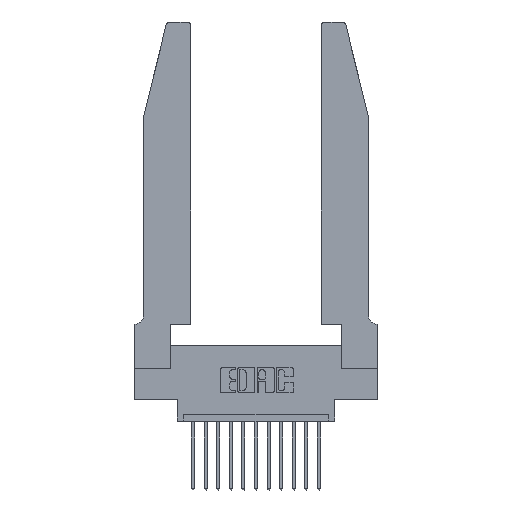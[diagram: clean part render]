
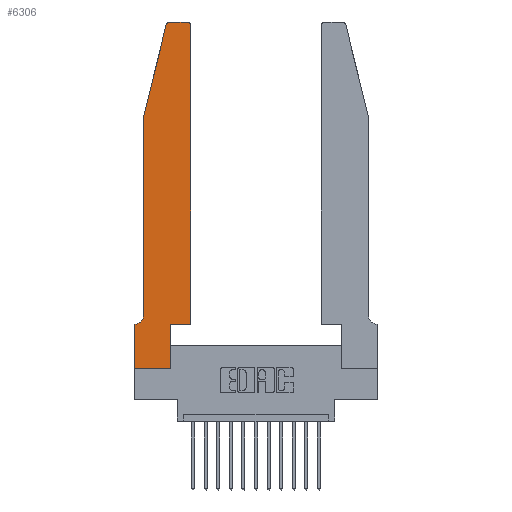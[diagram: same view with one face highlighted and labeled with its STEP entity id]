
A CAD part, top view. The second image highlights one B-rep face of the part: STEP entity #6306.
In plain terms, the highlighted planar face has unit normal (0, 0, 1).
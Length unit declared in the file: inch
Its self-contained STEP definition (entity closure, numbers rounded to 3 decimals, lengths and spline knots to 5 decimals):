
#153 = AXIS2_PLACEMENT_3D ( 'NONE', #14003, #10105, #600 ) ;
#323 = FACE_OUTER_BOUND ( 'NONE', #8452, .T. ) ;
#377 = ORIENTED_EDGE ( 'NONE', *, *, #4779, .T. ) ;
#395 = CARTESIAN_POINT ( 'NONE',  ( 0.0755, 0.35, 0.37 ) ) ;
#600 = DIRECTION ( 'NONE',  ( 1., 0., 0. ) ) ;
#689 = VECTOR ( 'NONE', #1014, 39.37008 ) ;
#958 = VERTEX_POINT ( 'NONE', #2403 ) ;
#1014 = DIRECTION ( 'NONE',  ( -1., 0., 0. ) ) ;
#1329 = LINE ( 'NONE', #4772, #14761 ) ;
#1339 = LINE ( 'NONE', #5969, #10384 ) ;
#1608 = CIRCLE ( 'NONE', #2971, 0.03 ) ;
#1632 = CARTESIAN_POINT ( 'NONE',  ( 0.2865, 0.35, 0.37 ) ) ;
#2056 = ORIENTED_EDGE ( 'NONE', *, *, #2181, .T. ) ;
#2110 = CIRCLE ( 'NONE', #12725, 0.03 ) ;
#2181 = EDGE_CURVE ( 'NONE', #13286, #14413, #14088, .T. ) ;
#2355 = CARTESIAN_POINT ( 'NONE',  ( 0.25487, 2.72718, 0.37 ) ) ;
#2403 = CARTESIAN_POINT ( 'NONE',  ( 0.0755, 2., 0.37 ) ) ;
#2713 = EDGE_CURVE ( 'NONE', #6629, #13286, #2110, .T. ) ;
#2945 = ORIENTED_EDGE ( 'NONE', *, *, #15720, .T. ) ;
#2971 = AXIS2_PLACEMENT_3D ( 'NONE', #3282, #15294, #15347 ) ;
#3141 = VERTEX_POINT ( 'NONE', #16645 ) ;
#3282 = CARTESIAN_POINT ( 'NONE',  ( 0.284, 2.72, 0.37 ) ) ;
#3353 = EDGE_CURVE ( 'NONE', #10981, #14024, #5868, .T. ) ;
#3660 = VERTEX_POINT ( 'NONE', #7959 ) ;
#3668 = CARTESIAN_POINT ( 'NONE',  ( 0.0055, 0.35, 0.37 ) ) ;
#3678 = DIRECTION ( 'NONE',  ( 1., 0., 0. ) ) ;
#4290 = DIRECTION ( 'NONE',  ( 0., 0., -1. ) ) ;
#4315 = LINE ( 'NONE', #15422, #9780 ) ;
#4403 = CARTESIAN_POINT ( 'NONE',  ( 0.0055, 0.42, 0.37 ) ) ;
#4507 = EDGE_CURVE ( 'NONE', #3660, #11042, #1329, .T. ) ;
#4772 = CARTESIAN_POINT ( 'NONE',  ( 0., 0., 0.37 ) ) ;
#4779 = EDGE_CURVE ( 'NONE', #14413, #10249, #1608, .T. ) ;
#4827 = DIRECTION ( 'NONE',  ( -0.239, -0.971, 0. ) ) ;
#4892 = CARTESIAN_POINT ( 'NONE',  ( 0.4505, 2.72, 0.37 ) ) ;
#5017 = CARTESIAN_POINT ( 'NONE',  ( 0.0755, 0.42, 0.37 ) ) ;
#5364 = CARTESIAN_POINT ( 'NONE',  ( 0.284, 2.75, 0.37 ) ) ;
#5475 = LINE ( 'NONE', #8338, #16787 ) ;
#5596 = DIRECTION ( 'NONE',  ( 0., 1., 0. ) ) ;
#5868 = LINE ( 'NONE', #1632, #7582 ) ;
#5969 = CARTESIAN_POINT ( 'NONE',  ( 0., 0., 0.37 ) ) ;
#6100 = PLANE ( 'NONE',  #153 ) ;
#6108 = DIRECTION ( 'NONE',  ( 0., -1., 0. ) ) ;
#6296 = CARTESIAN_POINT ( 'NONE',  ( 0.2605, 2.75, 0.37 ) ) ;
#6306 = ADVANCED_FACE ( 'NONE', ( #323 ), #6100, .T. ) ;
#6338 = ORIENTED_EDGE ( 'NONE', *, *, #11354, .T. ) ;
#6629 = VERTEX_POINT ( 'NONE', #4892 ) ;
#6937 = DIRECTION ( 'NONE',  ( -1., 0., 0. ) ) ;
#7026 = LINE ( 'NONE', #7997, #16649 ) ;
#7344 = EDGE_CURVE ( 'NONE', #14024, #3141, #7026, .T. ) ;
#7582 = VECTOR ( 'NONE', #15115, 39.37008 ) ;
#7584 = LINE ( 'NONE', #395, #8218 ) ;
#7959 = CARTESIAN_POINT ( 'NONE',  ( 0., 0.35, 0.37 ) ) ;
#7997 = CARTESIAN_POINT ( 'NONE',  ( 0.4505, 0.35, 0.37 ) ) ;
#8088 = CARTESIAN_POINT ( 'NONE',  ( 0.4205, 2.75, 0.37 ) ) ;
#8218 = VECTOR ( 'NONE', #15055, 39.37008 ) ;
#8338 = CARTESIAN_POINT ( 'NONE',  ( 0.4505, 0.35, 0.37 ) ) ;
#8452 = EDGE_LOOP ( 'NONE', ( #2056, #377, #6338, #14356, #17164, #15142, #10183, #15029, #12693, #14952, #2945, #16640 ) ) ;
#8518 = CARTESIAN_POINT ( 'NONE',  ( 0.2865, 0.35, 0.37 ) ) ;
#9210 = DIRECTION ( 'NONE',  ( 1., 0., 0. ) ) ;
#9258 = EDGE_CURVE ( 'NONE', #15383, #3660, #7584, .T. ) ;
#9780 = VECTOR ( 'NONE', #6108, 39.37008 ) ;
#10105 = DIRECTION ( 'NONE',  ( 0., 0., 1. ) ) ;
#10183 = ORIENTED_EDGE ( 'NONE', *, *, #4507, .T. ) ;
#10249 = VERTEX_POINT ( 'NONE', #2355 ) ;
#10359 = CARTESIAN_POINT ( 'NONE',  ( 0.4205, 2.72, 0.37 ) ) ;
#10384 = VECTOR ( 'NONE', #11734, 39.37008 ) ;
#10417 = DIRECTION ( 'NONE',  ( 0., 0., 1. ) ) ;
#10456 = EDGE_CURVE ( 'NONE', #14273, #15383, #12554, .T. ) ;
#10858 = CARTESIAN_POINT ( 'NONE',  ( 0.2865, 0., 0.37 ) ) ;
#10981 = VERTEX_POINT ( 'NONE', #10858 ) ;
#11042 = VERTEX_POINT ( 'NONE', #16146 ) ;
#11354 = EDGE_CURVE ( 'NONE', #10249, #958, #16711, .T. ) ;
#11734 = DIRECTION ( 'NONE',  ( 1., 0., 0. ) ) ;
#12554 = CIRCLE ( 'NONE', #14115, 0.07 ) ;
#12693 = ORIENTED_EDGE ( 'NONE', *, *, #3353, .T. ) ;
#12725 = AXIS2_PLACEMENT_3D ( 'NONE', #10359, #10417, #3678 ) ;
#12877 = DIRECTION ( 'NONE',  ( 0., -1., 0. ) ) ;
#13172 = VECTOR ( 'NONE', #4827, 39.37008 ) ;
#13286 = VERTEX_POINT ( 'NONE', #8088 ) ;
#13624 = EDGE_CURVE ( 'NONE', #958, #14273, #4315, .T. ) ;
#14003 = CARTESIAN_POINT ( 'NONE',  ( 0., 0.35, 0.37 ) ) ;
#14024 = VERTEX_POINT ( 'NONE', #8518 ) ;
#14088 = LINE ( 'NONE', #6296, #689 ) ;
#14115 = AXIS2_PLACEMENT_3D ( 'NONE', #4403, #4290, #6937 ) ;
#14235 = EDGE_CURVE ( 'NONE', #11042, #10981, #1339, .T. ) ;
#14273 = VERTEX_POINT ( 'NONE', #5017 ) ;
#14356 = ORIENTED_EDGE ( 'NONE', *, *, #13624, .T. ) ;
#14413 = VERTEX_POINT ( 'NONE', #5364 ) ;
#14761 = VECTOR ( 'NONE', #12877, 39.37008 ) ;
#14952 = ORIENTED_EDGE ( 'NONE', *, *, #7344, .T. ) ;
#15029 = ORIENTED_EDGE ( 'NONE', *, *, #14235, .T. ) ;
#15055 = DIRECTION ( 'NONE',  ( -1., 0., 0. ) ) ;
#15115 = DIRECTION ( 'NONE',  ( 0., 1., 0. ) ) ;
#15142 = ORIENTED_EDGE ( 'NONE', *, *, #9258, .T. ) ;
#15294 = DIRECTION ( 'NONE',  ( 0., 0., 1. ) ) ;
#15347 = DIRECTION ( 'NONE',  ( 1., 0., 0. ) ) ;
#15383 = VERTEX_POINT ( 'NONE', #3668 ) ;
#15422 = CARTESIAN_POINT ( 'NONE',  ( 0.0755, 2., 0.37 ) ) ;
#15550 = CARTESIAN_POINT ( 'NONE',  ( 0.0755, 2., 0.37 ) ) ;
#15720 = EDGE_CURVE ( 'NONE', #3141, #6629, #5475, .T. ) ;
#16146 = CARTESIAN_POINT ( 'NONE',  ( 0., 0., 0.37 ) ) ;
#16640 = ORIENTED_EDGE ( 'NONE', *, *, #2713, .T. ) ;
#16645 = CARTESIAN_POINT ( 'NONE',  ( 0.4505, 0.35, 0.37 ) ) ;
#16649 = VECTOR ( 'NONE', #9210, 39.37008 ) ;
#16711 = LINE ( 'NONE', #15550, #13172 ) ;
#16787 = VECTOR ( 'NONE', #5596, 39.37008 ) ;
#17164 = ORIENTED_EDGE ( 'NONE', *, *, #10456, .T. ) ;
